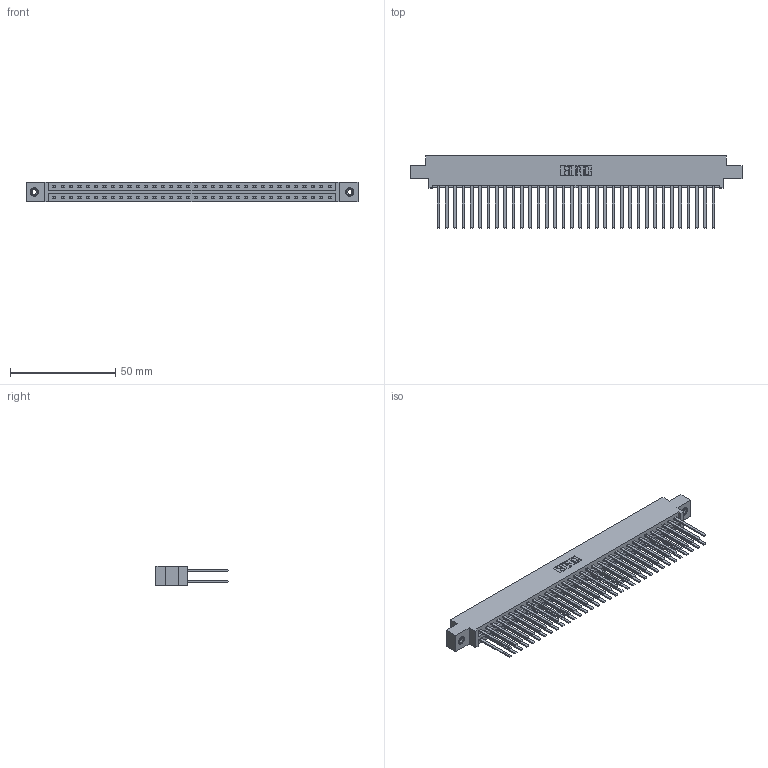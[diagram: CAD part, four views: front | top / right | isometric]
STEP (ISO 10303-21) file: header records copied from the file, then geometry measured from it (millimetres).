
FILE_DESCRIPTION (( 'STEP AP203' ), '1' );
FILE_NAME ('337-068-544-808.STEP', '2018-08-11T10:26:14', ( '' ), ( '' ), 'SwSTEP 2.0', 'SolidWorks 2016', '' );
FILE_SCHEMA (( 'CONFIG_CONTROL_DESIGN' ));
Length unit declared in the file: inch
Products named in the file (4): 337 Part_0.170 Offset - 0.156 Dia-TI; 345-292-001_345-293-144; 345-250-001_345-250-003-102; 337-068-544-808
Assembly tree (71 placements, depth 2):
  337-068-544-808
    337 Part_0.170 Offset - 0.156 Dia-TI
    345-292-001_345-293-144  x68
    345-250-001_345-250-003-102  x2
Bounding box: 157.73 x 34.3 x 9.4 mm (x, y, z)
Volume: 17346 mm3; surface area: 22777.7 mm2
Topology: 71 solids, 71 shells, 3442 faces, 10183 edges, 6690 vertices
Faces by surface type: plane 2418, cylinder 1008, cone 12, torus 4
Entity records: 28530 total; most frequent: CARTESIAN_POINT 4793, ORIENTED_EDGE 4722, DIRECTION 4119, EDGE_CURVE 2361, LINE 2217, VECTOR 2217, VERTEX_POINT 1568, AXIS2_PLACEMENT_3D 951
